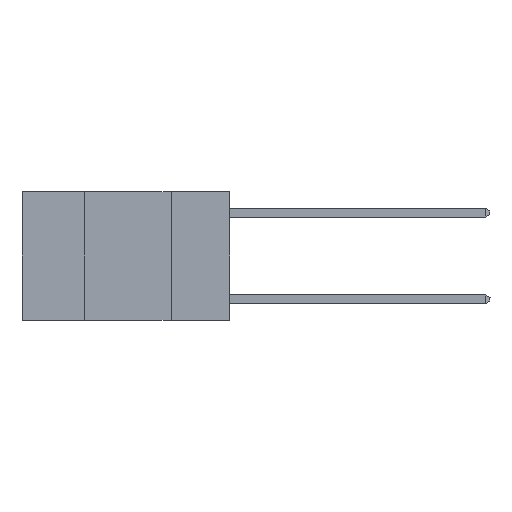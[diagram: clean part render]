
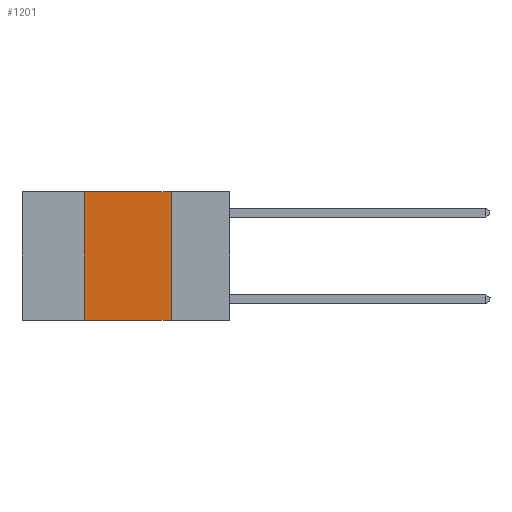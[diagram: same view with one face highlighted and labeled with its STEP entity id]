
A CAD part, left-side view. The second image highlights one B-rep face of the part: STEP entity #1201.
In plain terms, the highlighted planar face has unit normal (-1, 0, 0).
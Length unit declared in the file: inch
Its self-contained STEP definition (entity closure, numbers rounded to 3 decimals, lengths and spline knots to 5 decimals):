
#68 = CARTESIAN_POINT ( 'NONE',  ( 0., 0.6, 0. ) ) ;
#434 = ORIENTED_EDGE ( 'NONE', *, *, #4198, .F. ) ;
#1201 = ADVANCED_FACE ( 'NONE', ( #10492 ), #8362, .F. ) ;
#2530 = VERTEX_POINT ( 'NONE', #4167 ) ;
#2704 = DIRECTION ( 'NONE',  ( 0., -1., 0. ) ) ;
#2807 = AXIS2_PLACEMENT_3D ( 'NONE', #68, #7449, #5810 ) ;
#3341 = EDGE_CURVE ( 'NONE', #6369, #2530, #7921, .T. ) ;
#3367 = VERTEX_POINT ( 'NONE', #11486 ) ;
#3368 = VECTOR ( 'NONE', #2704, 39.37008 ) ;
#3997 = DIRECTION ( 'NONE',  ( 0., 0., 1. ) ) ;
#4167 = CARTESIAN_POINT ( 'NONE',  ( 0., 0.17, 0. ) ) ;
#4198 = EDGE_CURVE ( 'NONE', #2530, #6532, #7236, .T. ) ;
#4230 = LINE ( 'NONE', #5647, #10941 ) ;
#4475 = EDGE_CURVE ( 'NONE', #3367, #6369, #7092, .T. ) ;
#5647 = CARTESIAN_POINT ( 'NONE',  ( 0., 0.6, -0.37 ) ) ;
#5686 = DIRECTION ( 'NONE',  ( 0., -1., 0. ) ) ;
#5810 = DIRECTION ( 'NONE',  ( 0., 0., -1. ) ) ;
#6058 = CARTESIAN_POINT ( 'NONE',  ( 0., 0.42, 0. ) ) ;
#6369 = VERTEX_POINT ( 'NONE', #6058 ) ;
#6532 = VERTEX_POINT ( 'NONE', #9808 ) ;
#6564 = VECTOR ( 'NONE', #3997, 39.37008 ) ;
#6853 = ORIENTED_EDGE ( 'NONE', *, *, #3341, .F. ) ;
#7092 = LINE ( 'NONE', #10990, #6564 ) ;
#7236 = LINE ( 'NONE', #9774, #9360 ) ;
#7449 = DIRECTION ( 'NONE',  ( 1., 0., 0. ) ) ;
#7921 = LINE ( 'NONE', #11374, #3368 ) ;
#8362 = PLANE ( 'NONE',  #2807 ) ;
#9339 = ORIENTED_EDGE ( 'NONE', *, *, #10341, .T. ) ;
#9360 = VECTOR ( 'NONE', #9811, 39.37008 ) ;
#9598 = ORIENTED_EDGE ( 'NONE', *, *, #4475, .F. ) ;
#9774 = CARTESIAN_POINT ( 'NONE',  ( 0., 0.17, 0. ) ) ;
#9808 = CARTESIAN_POINT ( 'NONE',  ( 0., 0.17, -0.37 ) ) ;
#9811 = DIRECTION ( 'NONE',  ( 0., 0., -1. ) ) ;
#10341 = EDGE_CURVE ( 'NONE', #3367, #6532, #4230, .T. ) ;
#10354 = EDGE_LOOP ( 'NONE', ( #434, #6853, #9598, #9339 ) ) ;
#10492 = FACE_OUTER_BOUND ( 'NONE', #10354, .T. ) ;
#10941 = VECTOR ( 'NONE', #5686, 39.37008 ) ;
#10990 = CARTESIAN_POINT ( 'NONE',  ( 0., 0.42, 0. ) ) ;
#11374 = CARTESIAN_POINT ( 'NONE',  ( 0., 0.6, 0. ) ) ;
#11486 = CARTESIAN_POINT ( 'NONE',  ( 0., 0.42, -0.37 ) ) ;
